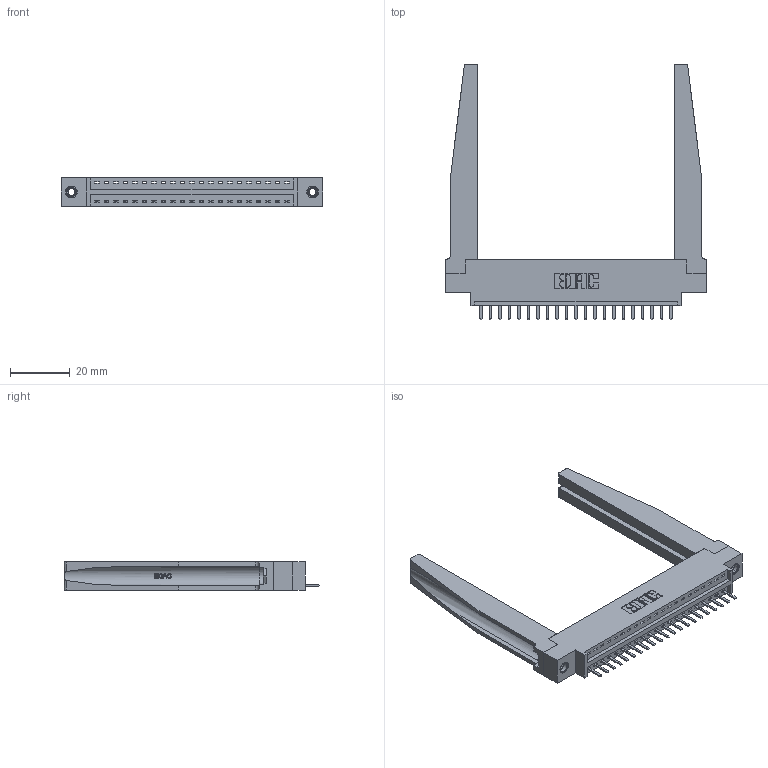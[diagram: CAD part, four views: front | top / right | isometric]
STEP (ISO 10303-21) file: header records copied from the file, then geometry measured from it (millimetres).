
FILE_DESCRIPTION (( 'STEP AP203' ), '1' );
FILE_NAME ('346-021-520-678.STEP', '2022-05-05T17:41:10', ( '' ), ( '' ), 'SwSTEP 2.0', 'SolidWorks 2020', '' );
FILE_SCHEMA (( 'CONFIG_CONTROL_DESIGN' ));
Length unit declared in the file: inch
Products named in the file (5): 346-021-520-678; 345-292-001_345-293-120; 346-220-078_345-220-078; 345-250-001_345-250-001-102; 346 Part_0.170 Offset - 0.156 Dia-TH
Assembly tree (26 placements, depth 2):
  346-021-520-678
    346 Part_0.170 Offset - 0.156 Dia-TH
    345-292-001_345-293-120  x21
    346-220-078_345-220-078  x2
    345-250-001_345-250-001-102  x2
Bounding box: 87.25 x 85.29 x 9.4 mm (x, y, z)
Volume: 14882.7 mm3; surface area: 16270.8 mm2
Topology: 26 solids, 26 shells, 1676 faces, 4849 edges, 3166 vertices
Faces by surface type: plane 1118, cylinder 506, bspline 36, cone 12, torus 4
Entity records: 21270 total; most frequent: CARTESIAN_POINT 4580, ORIENTED_EDGE 3410, DIRECTION 3037, EDGE_CURVE 1705, VECTOR 1391, LINE 1391, VERTEX_POINT 1128, AXIS2_PLACEMENT_3D 823
